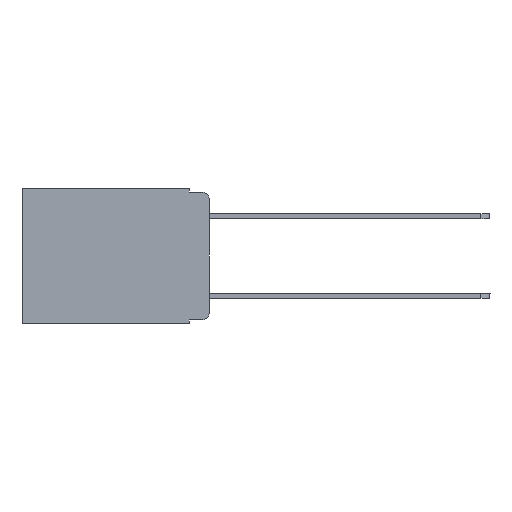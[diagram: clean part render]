
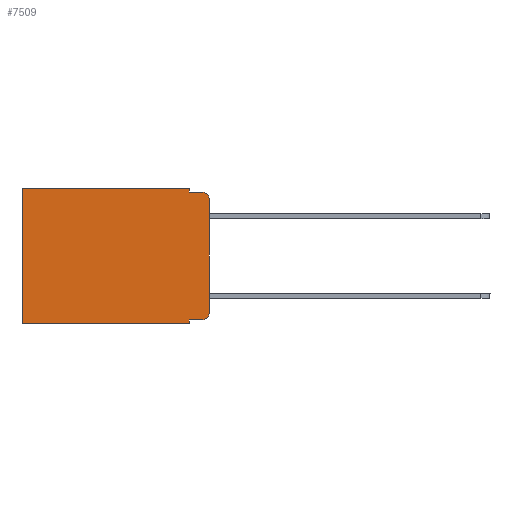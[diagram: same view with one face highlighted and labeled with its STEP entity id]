
A CAD part, left-side view. The second image highlights one B-rep face of the part: STEP entity #7509.
In plain terms, the highlighted planar face has unit normal (-1, 0, 0).
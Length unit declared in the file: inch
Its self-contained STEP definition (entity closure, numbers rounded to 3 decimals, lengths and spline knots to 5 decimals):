
#149 = LINE ( 'NONE', #4770, #2588 ) ;
#321 = DIRECTION ( 'NONE',  ( 1., 0., 0. ) ) ;
#361 = ORIENTED_EDGE ( 'NONE', *, *, #2965, .F. ) ;
#387 = VERTEX_POINT ( 'NONE', #4491 ) ;
#472 = DIRECTION ( 'NONE',  ( -1., 0., 0. ) ) ;
#1016 = VERTEX_POINT ( 'NONE', #12164 ) ;
#1041 = DIRECTION ( 'NONE',  ( -1., 0., 0. ) ) ;
#1082 = CARTESIAN_POINT ( 'NONE',  ( 0.298, 0.051, 0. ) ) ;
#1118 = ORIENTED_EDGE ( 'NONE', *, *, #7711, .T. ) ;
#1173 = VECTOR ( 'NONE', #9530, 39.37008 ) ;
#1345 = CARTESIAN_POINT ( 'NONE',  ( 0.298, 0., -0.313 ) ) ;
#1442 = CARTESIAN_POINT ( 'NONE',  ( 0.298, 0., 0. ) ) ;
#1545 = DIRECTION ( 'NONE',  ( 0., -1., 0. ) ) ;
#1551 = LINE ( 'NONE', #10004, #8086 ) ;
#1598 = VECTOR ( 'NONE', #12705, 39.37008 ) ;
#1697 = EDGE_CURVE ( 'NONE', #5739, #13211, #2961, .T. ) ;
#1871 = LINE ( 'NONE', #4297, #1598 ) ;
#1875 = VERTEX_POINT ( 'NONE', #14710 ) ;
#2268 = CARTESIAN_POINT ( 'NONE',  ( 0.298, 0.051, -0.01 ) ) ;
#2311 = VERTEX_POINT ( 'NONE', #11134 ) ;
#2492 = ORIENTED_EDGE ( 'NONE', *, *, #8898, .F. ) ;
#2588 = VECTOR ( 'NONE', #6127, 39.37008 ) ;
#2690 = PLANE ( 'NONE',  #10363 ) ;
#2961 = CIRCLE ( 'NONE', #5466, 0.02 ) ;
#2965 = EDGE_CURVE ( 'NONE', #1016, #13374, #13932, .T. ) ;
#4297 = CARTESIAN_POINT ( 'NONE',  ( 0.298, 0., -0.343 ) ) ;
#4373 = LINE ( 'NONE', #1082, #1173 ) ;
#4420 = LINE ( 'NONE', #8808, #15455 ) ;
#4491 = CARTESIAN_POINT ( 'NONE',  ( 0.298, 0.473, -0.343 ) ) ;
#4545 = AXIS2_PLACEMENT_3D ( 'NONE', #15001, #472, #7882 ) ;
#4770 = CARTESIAN_POINT ( 'NONE',  ( 0.298, 0.473, 0. ) ) ;
#5296 = EDGE_CURVE ( 'NONE', #5321, #6589, #4373, .T. ) ;
#5304 = VECTOR ( 'NONE', #5471, 39.37008 ) ;
#5321 = VERTEX_POINT ( 'NONE', #9838 ) ;
#5466 = AXIS2_PLACEMENT_3D ( 'NONE', #5935, #1041, #15424 ) ;
#5471 = DIRECTION ( 'NONE',  ( 0., 0., -1. ) ) ;
#5739 = VERTEX_POINT ( 'NONE', #11963 ) ;
#5740 = CARTESIAN_POINT ( 'NONE',  ( 0.298, 0.02, -0.01 ) ) ;
#5935 = CARTESIAN_POINT ( 'NONE',  ( 0.298, 0.02, -0.03 ) ) ;
#6127 = DIRECTION ( 'NONE',  ( 0., 0., -1. ) ) ;
#6589 = VERTEX_POINT ( 'NONE', #2268 ) ;
#6833 = EDGE_CURVE ( 'NONE', #1016, #1875, #1551, .T. ) ;
#6899 = CARTESIAN_POINT ( 'NONE',  ( 0.298, 0., 0. ) ) ;
#7289 = LINE ( 'NONE', #1442, #14209 ) ;
#7348 = EDGE_CURVE ( 'NONE', #5321, #2311, #11558, .T. ) ;
#7454 = VERTEX_POINT ( 'NONE', #1345 ) ;
#7509 = ADVANCED_FACE ( 'NONE', ( #10995 ), #2690, .F. ) ;
#7711 = EDGE_CURVE ( 'NONE', #1875, #7454, #11386, .T. ) ;
#7882 = DIRECTION ( 'NONE',  ( 0., 0., -1. ) ) ;
#8086 = VECTOR ( 'NONE', #10240, 39.37008 ) ;
#8218 = CARTESIAN_POINT ( 'NONE',  ( 0.298, 0.051, -0.343 ) ) ;
#8604 = VECTOR ( 'NONE', #13000, 39.37008 ) ;
#8780 = EDGE_CURVE ( 'NONE', #2311, #387, #149, .T. ) ;
#8808 = CARTESIAN_POINT ( 'NONE',  ( 0.298, 0.051, -0.01 ) ) ;
#8898 = EDGE_CURVE ( 'NONE', #6589, #13211, #4420, .T. ) ;
#9116 = EDGE_CURVE ( 'NONE', #5739, #7454, #7289, .T. ) ;
#9419 = DIRECTION ( 'NONE',  ( 0., 0., -1. ) ) ;
#9465 = ORIENTED_EDGE ( 'NONE', *, *, #11024, .F. ) ;
#9514 = ORIENTED_EDGE ( 'NONE', *, *, #5296, .F. ) ;
#9530 = DIRECTION ( 'NONE',  ( 0., 0., -1. ) ) ;
#9838 = CARTESIAN_POINT ( 'NONE',  ( 0.298, 0.051, 0. ) ) ;
#10004 = CARTESIAN_POINT ( 'NONE',  ( 0.298, 0.051, -0.333 ) ) ;
#10110 = ORIENTED_EDGE ( 'NONE', *, *, #7348, .T. ) ;
#10240 = DIRECTION ( 'NONE',  ( 0., -1., 0. ) ) ;
#10363 = AXIS2_PLACEMENT_3D ( 'NONE', #13083, #321, #9419 ) ;
#10924 = DIRECTION ( 'NONE',  ( 0., 0., -1. ) ) ;
#10995 = FACE_OUTER_BOUND ( 'NONE', #11892, .T. ) ;
#11024 = EDGE_CURVE ( 'NONE', #13374, #387, #1871, .T. ) ;
#11110 = ORIENTED_EDGE ( 'NONE', *, *, #1697, .T. ) ;
#11134 = CARTESIAN_POINT ( 'NONE',  ( 0.298, 0.473, 0. ) ) ;
#11386 = CIRCLE ( 'NONE', #4545, 0.02 ) ;
#11558 = LINE ( 'NONE', #6899, #8604 ) ;
#11579 = ORIENTED_EDGE ( 'NONE', *, *, #6833, .T. ) ;
#11892 = EDGE_LOOP ( 'NONE', ( #12798, #11110, #2492, #9514, #10110, #13650, #9465, #361, #11579, #1118 ) ) ;
#11963 = CARTESIAN_POINT ( 'NONE',  ( 0.298, 0., -0.03 ) ) ;
#12164 = CARTESIAN_POINT ( 'NONE',  ( 0.298, 0.051, -0.333 ) ) ;
#12705 = DIRECTION ( 'NONE',  ( 0., 1., 0. ) ) ;
#12798 = ORIENTED_EDGE ( 'NONE', *, *, #9116, .F. ) ;
#13000 = DIRECTION ( 'NONE',  ( 0., 1., 0. ) ) ;
#13083 = CARTESIAN_POINT ( 'NONE',  ( 0.298, 0., 0. ) ) ;
#13211 = VERTEX_POINT ( 'NONE', #5740 ) ;
#13374 = VERTEX_POINT ( 'NONE', #8218 ) ;
#13650 = ORIENTED_EDGE ( 'NONE', *, *, #8780, .T. ) ;
#13932 = LINE ( 'NONE', #15121, #5304 ) ;
#14209 = VECTOR ( 'NONE', #10924, 39.37008 ) ;
#14710 = CARTESIAN_POINT ( 'NONE',  ( 0.298, 0.02, -0.333 ) ) ;
#15001 = CARTESIAN_POINT ( 'NONE',  ( 0.298, 0.02, -0.313 ) ) ;
#15121 = CARTESIAN_POINT ( 'NONE',  ( 0.298, 0.051, 0. ) ) ;
#15424 = DIRECTION ( 'NONE',  ( 0., 0., -1. ) ) ;
#15455 = VECTOR ( 'NONE', #1545, 39.37008 ) ;
